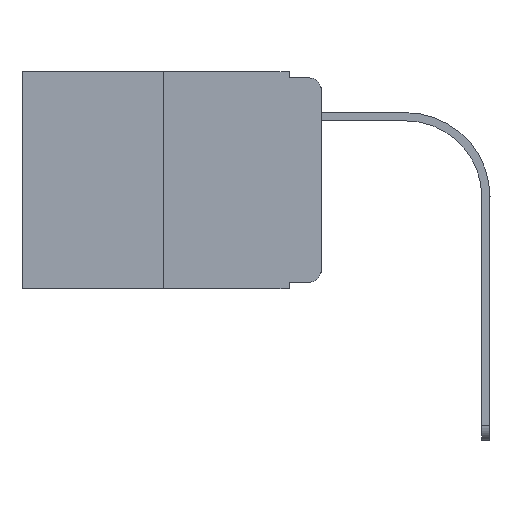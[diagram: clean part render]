
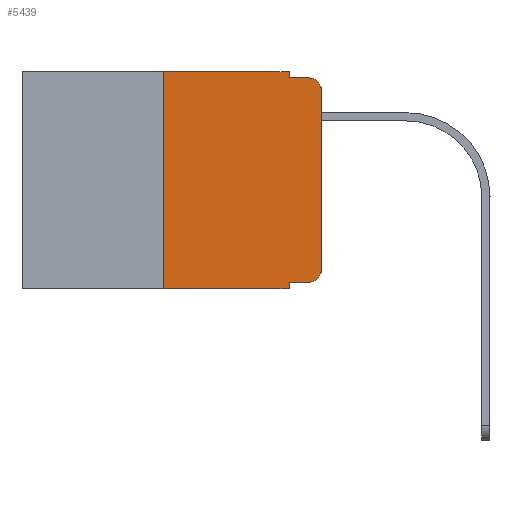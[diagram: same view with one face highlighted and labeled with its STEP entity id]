
A CAD part, left-side view. The second image highlights one B-rep face of the part: STEP entity #5439.
In plain terms, the highlighted planar face has unit normal (-1, 0, 0).
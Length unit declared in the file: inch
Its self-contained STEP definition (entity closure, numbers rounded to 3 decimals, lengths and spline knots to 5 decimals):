
#95 = VERTEX_POINT ( 'NONE', #9026 ) ;
#168 = CARTESIAN_POINT ( 'NONE',  ( 0., 0.473, 0. ) ) ;
#546 = CARTESIAN_POINT ( 'NONE',  ( 0., 0.051, -0.01 ) ) ;
#1418 = VERTEX_POINT ( 'NONE', #20448 ) ;
#1569 = ORIENTED_EDGE ( 'NONE', *, *, #20995, .F. ) ;
#1943 = CARTESIAN_POINT ( 'NONE',  ( 0., 0.02, -0.01 ) ) ;
#2027 = VERTEX_POINT ( 'NONE', #546 ) ;
#2423 = LINE ( 'NONE', #11411, #16406 ) ;
#2704 = EDGE_CURVE ( 'NONE', #9855, #7858, #18032, .T. ) ;
#2721 = CARTESIAN_POINT ( 'NONE',  ( 0., 0., -0.03 ) ) ;
#3063 = EDGE_CURVE ( 'NONE', #3411, #95, #12858, .T. ) ;
#3269 = DIRECTION ( 'NONE',  ( 0., 0., -1. ) ) ;
#3287 = VECTOR ( 'NONE', #17267, 39.37008 ) ;
#3411 = VERTEX_POINT ( 'NONE', #23710 ) ;
#3488 = DIRECTION ( 'NONE',  ( 0., 0., -1. ) ) ;
#3781 = ORIENTED_EDGE ( 'NONE', *, *, #17166, .T. ) ;
#3806 = DIRECTION ( 'NONE',  ( -1., 0., 0. ) ) ;
#4021 = LINE ( 'NONE', #7899, #3287 ) ;
#4066 = VERTEX_POINT ( 'NONE', #14972 ) ;
#4080 = AXIS2_PLACEMENT_3D ( 'NONE', #168, #12831, #3488 ) ;
#4528 = EDGE_CURVE ( 'NONE', #95, #21544, #4021, .T. ) ;
#5070 = CARTESIAN_POINT ( 'NONE',  ( 0., 0.02, -0.313 ) ) ;
#5080 = ORIENTED_EDGE ( 'NONE', *, *, #12975, .T. ) ;
#5439 = ADVANCED_FACE ( 'NONE', ( #16847 ), #5895, .F. ) ;
#5895 = PLANE ( 'NONE',  #4080 ) ;
#6027 = ORIENTED_EDGE ( 'NONE', *, *, #23123, .T. ) ;
#6485 = DIRECTION ( 'NONE',  ( 0., 0., 1. ) ) ;
#6630 = ORIENTED_EDGE ( 'NONE', *, *, #10537, .F. ) ;
#6836 = CARTESIAN_POINT ( 'NONE',  ( 0., 0.25, 0. ) ) ;
#7679 = DIRECTION ( 'NONE',  ( 0., 0., -1. ) ) ;
#7730 = AXIS2_PLACEMENT_3D ( 'NONE', #13384, #3806, #7679 ) ;
#7858 = VERTEX_POINT ( 'NONE', #13866 ) ;
#7899 = CARTESIAN_POINT ( 'NONE',  ( 0., 0., 0. ) ) ;
#8739 = VECTOR ( 'NONE', #13894, 39.37008 ) ;
#9026 = CARTESIAN_POINT ( 'NONE',  ( 0., 0., -0.313 ) ) ;
#9855 = VERTEX_POINT ( 'NONE', #22850 ) ;
#9955 = ORIENTED_EDGE ( 'NONE', *, *, #4528, .T. ) ;
#10537 = EDGE_CURVE ( 'NONE', #20103, #1418, #12295, .T. ) ;
#10656 = ORIENTED_EDGE ( 'NONE', *, *, #3063, .T. ) ;
#11411 = CARTESIAN_POINT ( 'NONE',  ( 0., 0.051, -0.333 ) ) ;
#11591 = CARTESIAN_POINT ( 'NONE',  ( 0., 0.473, 0. ) ) ;
#11935 = EDGE_CURVE ( 'NONE', #4066, #2027, #14477, .T. ) ;
#12295 = LINE ( 'NONE', #19738, #8739 ) ;
#12342 = VECTOR ( 'NONE', #14715, 39.37008 ) ;
#12829 = ORIENTED_EDGE ( 'NONE', *, *, #16802, .F. ) ;
#12831 = DIRECTION ( 'NONE',  ( 1., 0., 0. ) ) ;
#12858 = CIRCLE ( 'NONE', #14410, 0.02 ) ;
#12975 = EDGE_CURVE ( 'NONE', #9855, #1418, #24005, .T. ) ;
#13384 = CARTESIAN_POINT ( 'NONE',  ( 0., 0.02, -0.03 ) ) ;
#13866 = CARTESIAN_POINT ( 'NONE',  ( 0., 0.25, 0. ) ) ;
#13894 = DIRECTION ( 'NONE',  ( 0., 0., -1. ) ) ;
#14410 = AXIS2_PLACEMENT_3D ( 'NONE', #5070, #16273, #3269 ) ;
#14477 = LINE ( 'NONE', #18270, #16958 ) ;
#14715 = DIRECTION ( 'NONE',  ( 0., -1., 0. ) ) ;
#14842 = DIRECTION ( 'NONE',  ( 0., 0., -1. ) ) ;
#14972 = CARTESIAN_POINT ( 'NONE',  ( 0., 0.051, 0. ) ) ;
#15180 = CARTESIAN_POINT ( 'NONE',  ( 0., 0.051, -0.333 ) ) ;
#15199 = EDGE_LOOP ( 'NONE', ( #9955, #6027, #1569, #21772, #12829, #21236, #5080, #6630, #3781, #10656 ) ) ;
#15475 = CIRCLE ( 'NONE', #7730, 0.02 ) ;
#16273 = DIRECTION ( 'NONE',  ( -1., 0., 0. ) ) ;
#16406 = VECTOR ( 'NONE', #22543, 39.37008 ) ;
#16659 = CARTESIAN_POINT ( 'NONE',  ( 0., 0.051, -0.01 ) ) ;
#16802 = EDGE_CURVE ( 'NONE', #7858, #4066, #22833, .T. ) ;
#16847 = FACE_OUTER_BOUND ( 'NONE', #15199, .T. ) ;
#16958 = VECTOR ( 'NONE', #14842, 39.37008 ) ;
#17089 = VECTOR ( 'NONE', #6485, 39.37008 ) ;
#17166 = EDGE_CURVE ( 'NONE', #20103, #3411, #2423, .T. ) ;
#17194 = DIRECTION ( 'NONE',  ( 0., -1., 0. ) ) ;
#17267 = DIRECTION ( 'NONE',  ( 0., 0., 1. ) ) ;
#18032 = LINE ( 'NONE', #6836, #17089 ) ;
#18270 = CARTESIAN_POINT ( 'NONE',  ( 0., 0.051, 0. ) ) ;
#18725 = DIRECTION ( 'NONE',  ( 0., -1., 0. ) ) ;
#18742 = CARTESIAN_POINT ( 'NONE',  ( 0., 0.473, -0.343 ) ) ;
#19366 = VECTOR ( 'NONE', #18725, 39.37008 ) ;
#19738 = CARTESIAN_POINT ( 'NONE',  ( 0., 0.051, 0. ) ) ;
#20103 = VERTEX_POINT ( 'NONE', #15180 ) ;
#20448 = CARTESIAN_POINT ( 'NONE',  ( 0., 0.051, -0.343 ) ) ;
#20562 = VERTEX_POINT ( 'NONE', #1943 ) ;
#20995 = EDGE_CURVE ( 'NONE', #2027, #20562, #23988, .T. ) ;
#21236 = ORIENTED_EDGE ( 'NONE', *, *, #2704, .F. ) ;
#21474 = VECTOR ( 'NONE', #17194, 39.37008 ) ;
#21544 = VERTEX_POINT ( 'NONE', #2721 ) ;
#21772 = ORIENTED_EDGE ( 'NONE', *, *, #11935, .F. ) ;
#22543 = DIRECTION ( 'NONE',  ( 0., -1., 0. ) ) ;
#22833 = LINE ( 'NONE', #11591, #21474 ) ;
#22850 = CARTESIAN_POINT ( 'NONE',  ( 0., 0.25, -0.343 ) ) ;
#23123 = EDGE_CURVE ( 'NONE', #21544, #20562, #15475, .T. ) ;
#23710 = CARTESIAN_POINT ( 'NONE',  ( 0., 0.02, -0.333 ) ) ;
#23988 = LINE ( 'NONE', #16659, #19366 ) ;
#24005 = LINE ( 'NONE', #18742, #12342 ) ;
